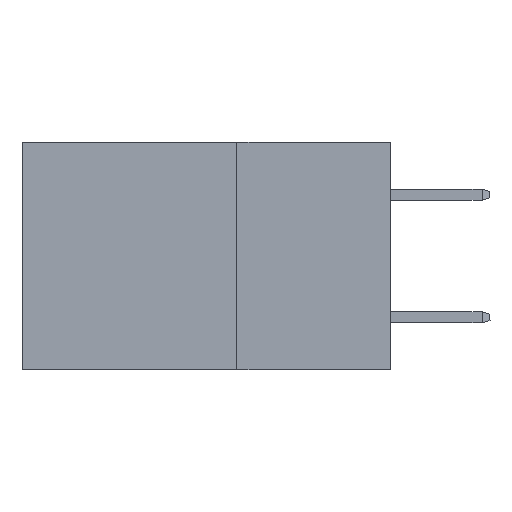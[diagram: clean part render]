
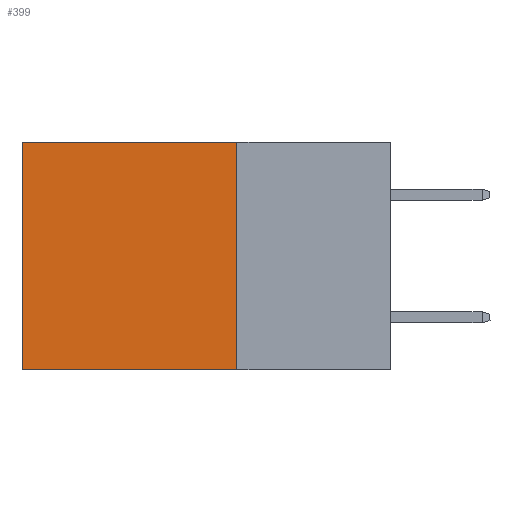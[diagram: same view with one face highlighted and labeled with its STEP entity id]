
A CAD part, left-side view. The second image highlights one B-rep face of the part: STEP entity #399.
In plain terms, the highlighted planar face has unit normal (-1, 0, 0).
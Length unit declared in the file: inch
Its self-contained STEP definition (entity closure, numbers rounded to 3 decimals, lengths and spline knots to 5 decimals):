
#95 = EDGE_CURVE ( 'NONE', #5697, #196, #7176, .T. ) ;
#196 = VERTEX_POINT ( 'NONE', #9677 ) ;
#375 = CARTESIAN_POINT ( 'NONE',  ( 0.2875, 0.25, -0.37 ) ) ;
#399 = ADVANCED_FACE ( 'NONE', ( #8022 ), #9107, .F. ) ;
#813 = LINE ( 'NONE', #5185, #13160 ) ;
#954 = CARTESIAN_POINT ( 'NONE',  ( 0.2875, 0.25, 0. ) ) ;
#1831 = DIRECTION ( 'NONE',  ( 0., 0., -1. ) ) ;
#1834 = EDGE_CURVE ( 'NONE', #3701, #5697, #9514, .T. ) ;
#2193 = ORIENTED_EDGE ( 'NONE', *, *, #1834, .T. ) ;
#2337 = ORIENTED_EDGE ( 'NONE', *, *, #6508, .F. ) ;
#2414 = DIRECTION ( 'NONE',  ( 0., 0., -1. ) ) ;
#2465 = CARTESIAN_POINT ( 'NONE',  ( 0.2875, 0.25, 0. ) ) ;
#3068 = DIRECTION ( 'NONE',  ( 0., 1., 0. ) ) ;
#3248 = EDGE_LOOP ( 'NONE', ( #11737, #2337, #13332, #2193 ) ) ;
#3668 = VECTOR ( 'NONE', #1831, 39.37008 ) ;
#3701 = VERTEX_POINT ( 'NONE', #2465 ) ;
#4115 = VECTOR ( 'NONE', #13821, 39.37008 ) ;
#4214 = CARTESIAN_POINT ( 'NONE',  ( 0.2875, 0.6, 0. ) ) ;
#4483 = CARTESIAN_POINT ( 'NONE',  ( 0.2875, 0.25, 0. ) ) ;
#4533 = LINE ( 'NONE', #13224, #8651 ) ;
#5185 = CARTESIAN_POINT ( 'NONE',  ( 0.2875, 0.25, -0.37 ) ) ;
#5697 = VERTEX_POINT ( 'NONE', #4214 ) ;
#6508 = EDGE_CURVE ( 'NONE', #6721, #196, #813, .T. ) ;
#6721 = VERTEX_POINT ( 'NONE', #375 ) ;
#6741 = EDGE_CURVE ( 'NONE', #3701, #6721, #4533, .T. ) ;
#7176 = LINE ( 'NONE', #11369, #3668 ) ;
#8022 = FACE_OUTER_BOUND ( 'NONE', #3248, .T. ) ;
#8651 = VECTOR ( 'NONE', #2414, 39.37008 ) ;
#8809 = DIRECTION ( 'NONE',  ( 0., 0., -1. ) ) ;
#9107 = PLANE ( 'NONE',  #11784 ) ;
#9514 = LINE ( 'NONE', #954, #4115 ) ;
#9677 = CARTESIAN_POINT ( 'NONE',  ( 0.2875, 0.6, -0.37 ) ) ;
#11068 = DIRECTION ( 'NONE',  ( 1., 0., 0. ) ) ;
#11369 = CARTESIAN_POINT ( 'NONE',  ( 0.2875, 0.6, 0. ) ) ;
#11737 = ORIENTED_EDGE ( 'NONE', *, *, #95, .T. ) ;
#11784 = AXIS2_PLACEMENT_3D ( 'NONE', #4483, #11068, #8809 ) ;
#13160 = VECTOR ( 'NONE', #3068, 39.37008 ) ;
#13224 = CARTESIAN_POINT ( 'NONE',  ( 0.2875, 0.25, 0. ) ) ;
#13332 = ORIENTED_EDGE ( 'NONE', *, *, #6741, .F. ) ;
#13821 = DIRECTION ( 'NONE',  ( 0., 1., 0. ) ) ;
